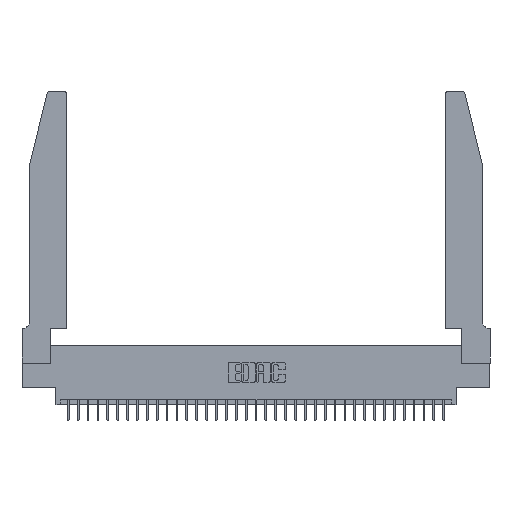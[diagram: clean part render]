
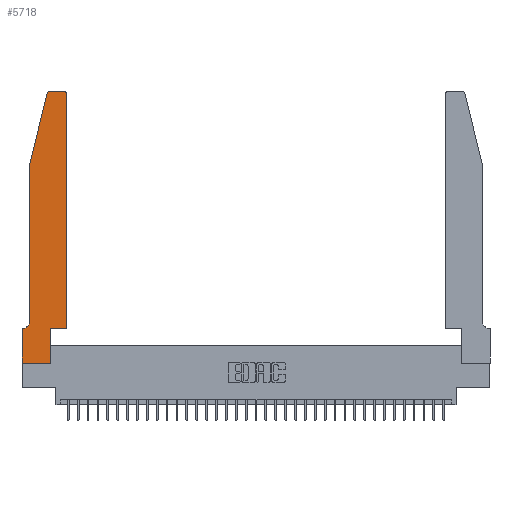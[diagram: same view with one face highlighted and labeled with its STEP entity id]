
A CAD part, top view. The second image highlights one B-rep face of the part: STEP entity #5718.
In plain terms, the highlighted planar face has unit normal (0, 0, 1).
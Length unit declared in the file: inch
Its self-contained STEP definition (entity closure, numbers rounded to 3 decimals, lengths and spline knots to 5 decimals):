
#95 = EDGE_CURVE ( 'NONE', #31149, #14235, #27200, .T. ) ;
#813 = CARTESIAN_POINT ( 'NONE',  ( 0., 0.35, 0.37 ) ) ;
#978 = CARTESIAN_POINT ( 'NONE',  ( 0.2865, 0.35, 0.37 ) ) ;
#1143 = VERTEX_POINT ( 'NONE', #2586 ) ;
#1711 = VECTOR ( 'NONE', #28622, 39.37008 ) ;
#2111 = CARTESIAN_POINT ( 'NONE',  ( 0.0755, 0.42, 0.37 ) ) ;
#2343 = CARTESIAN_POINT ( 'NONE',  ( 0., 0., 0.37 ) ) ;
#2586 = CARTESIAN_POINT ( 'NONE',  ( 0.4205, 2.75, 0.37 ) ) ;
#2658 = AXIS2_PLACEMENT_3D ( 'NONE', #31968, #15398, #34719 ) ;
#3021 = CARTESIAN_POINT ( 'NONE',  ( 0.4505, 0.35, 0.37 ) ) ;
#4048 = CARTESIAN_POINT ( 'NONE',  ( 0., 0.35, 0.37 ) ) ;
#4121 = ORIENTED_EDGE ( 'NONE', *, *, #35960, .T. ) ;
#4205 = VERTEX_POINT ( 'NONE', #33162 ) ;
#4545 = AXIS2_PLACEMENT_3D ( 'NONE', #4048, #9674, #29089 ) ;
#5190 = EDGE_CURVE ( 'NONE', #6918, #26862, #29895, .T. ) ;
#5718 = ADVANCED_FACE ( 'NONE', ( #28145 ), #23431, .T. ) ;
#5786 = VECTOR ( 'NONE', #21912, 39.37008 ) ;
#5809 = CARTESIAN_POINT ( 'NONE',  ( 0.4205, 2.72, 0.37 ) ) ;
#5863 = LINE ( 'NONE', #28262, #19833 ) ;
#6918 = VERTEX_POINT ( 'NONE', #2111 ) ;
#7825 = CIRCLE ( 'NONE', #2658, 0.03 ) ;
#8648 = DIRECTION ( 'NONE',  ( 1., 0., 0. ) ) ;
#8929 = LINE ( 'NONE', #9425, #29325 ) ;
#9186 = LINE ( 'NONE', #15319, #24863 ) ;
#9215 = CARTESIAN_POINT ( 'NONE',  ( 0., 0., 0.37 ) ) ;
#9425 = CARTESIAN_POINT ( 'NONE',  ( 0.4505, 0.35, 0.37 ) ) ;
#9674 = DIRECTION ( 'NONE',  ( 0., 0., 1. ) ) ;
#10870 = ORIENTED_EDGE ( 'NONE', *, *, #11016, .T. ) ;
#11016 = EDGE_CURVE ( 'NONE', #16986, #30710, #35275, .T. ) ;
#11626 = LINE ( 'NONE', #18405, #32845 ) ;
#12238 = DIRECTION ( 'NONE',  ( 1., 0., 0. ) ) ;
#12342 = EDGE_CURVE ( 'NONE', #30710, #21502, #28571, .T. ) ;
#12428 = VECTOR ( 'NONE', #19741, 39.37008 ) ;
#12809 = ORIENTED_EDGE ( 'NONE', *, *, #17404, .T. ) ;
#13432 = CARTESIAN_POINT ( 'NONE',  ( 0.0755, 2., 0.37 ) ) ;
#13555 = CARTESIAN_POINT ( 'NONE',  ( 0.25487, 2.72718, 0.37 ) ) ;
#13995 = ORIENTED_EDGE ( 'NONE', *, *, #18791, .T. ) ;
#14128 = ORIENTED_EDGE ( 'NONE', *, *, #95, .T. ) ;
#14235 = VERTEX_POINT ( 'NONE', #31734 ) ;
#14245 = ORIENTED_EDGE ( 'NONE', *, *, #12342, .T. ) ;
#14613 = CARTESIAN_POINT ( 'NONE',  ( 0.2865, 0., 0.37 ) ) ;
#14697 = VECTOR ( 'NONE', #28741, 39.37008 ) ;
#14736 = ORIENTED_EDGE ( 'NONE', *, *, #26750, .T. ) ;
#15319 = CARTESIAN_POINT ( 'NONE',  ( 0.0755, 0.35, 0.37 ) ) ;
#15398 = DIRECTION ( 'NONE',  ( 0., 0., 1. ) ) ;
#15996 = CARTESIAN_POINT ( 'NONE',  ( 0.0055, 0.35, 0.37 ) ) ;
#16068 = CARTESIAN_POINT ( 'NONE',  ( 0.0055, 0.42, 0.37 ) ) ;
#16353 = CARTESIAN_POINT ( 'NONE',  ( 0.2865, 0.35, 0.37 ) ) ;
#16740 = EDGE_CURVE ( 'NONE', #26862, #30041, #9186, .T. ) ;
#16756 = AXIS2_PLACEMENT_3D ( 'NONE', #5809, #25304, #8648 ) ;
#16986 = VERTEX_POINT ( 'NONE', #2343 ) ;
#17404 = EDGE_CURVE ( 'NONE', #4205, #26925, #7825, .T. ) ;
#18153 = LINE ( 'NONE', #18286, #32005 ) ;
#18220 = DIRECTION ( 'NONE',  ( -1., 0., 0. ) ) ;
#18286 = CARTESIAN_POINT ( 'NONE',  ( 0.2605, 2.75, 0.37 ) ) ;
#18405 = CARTESIAN_POINT ( 'NONE',  ( 0.0755, 2., 0.37 ) ) ;
#18791 = EDGE_CURVE ( 'NONE', #14235, #1143, #33930, .T. ) ;
#18844 = DIRECTION ( 'NONE',  ( -1., 0., 0. ) ) ;
#18991 = CARTESIAN_POINT ( 'NONE',  ( 0., 0., 0.37 ) ) ;
#19211 = CARTESIAN_POINT ( 'NONE',  ( 0.4505, 0.35, 0.37 ) ) ;
#19741 = DIRECTION ( 'NONE',  ( 0., 1., 0. ) ) ;
#19833 = VECTOR ( 'NONE', #31034, 39.37008 ) ;
#21074 = DIRECTION ( 'NONE',  ( -1., 0., 0. ) ) ;
#21502 = VERTEX_POINT ( 'NONE', #16353 ) ;
#21912 = DIRECTION ( 'NONE',  ( 1., 0., 0. ) ) ;
#23431 = PLANE ( 'NONE',  #4545 ) ;
#24863 = VECTOR ( 'NONE', #18220, 39.37008 ) ;
#25262 = ORIENTED_EDGE ( 'NONE', *, *, #5190, .T. ) ;
#25304 = DIRECTION ( 'NONE',  ( 0., 0., 1. ) ) ;
#26750 = EDGE_CURVE ( 'NONE', #1143, #4205, #18153, .T. ) ;
#26862 = VERTEX_POINT ( 'NONE', #15996 ) ;
#26925 = VERTEX_POINT ( 'NONE', #13555 ) ;
#27200 = LINE ( 'NONE', #3021, #12428 ) ;
#28145 = FACE_OUTER_BOUND ( 'NONE', #33142, .T. ) ;
#28262 = CARTESIAN_POINT ( 'NONE',  ( 0.0755, 2., 0.37 ) ) ;
#28571 = LINE ( 'NONE', #978, #14697 ) ;
#28622 = DIRECTION ( 'NONE',  ( 0., -1., 0. ) ) ;
#28741 = DIRECTION ( 'NONE',  ( 0., 1., 0. ) ) ;
#28819 = VERTEX_POINT ( 'NONE', #13432 ) ;
#28957 = ORIENTED_EDGE ( 'NONE', *, *, #34932, .T. ) ;
#29077 = AXIS2_PLACEMENT_3D ( 'NONE', #16068, #35370, #18844 ) ;
#29089 = DIRECTION ( 'NONE',  ( 1., 0., 0. ) ) ;
#29325 = VECTOR ( 'NONE', #12238, 39.37008 ) ;
#29895 = CIRCLE ( 'NONE', #29077, 0.07 ) ;
#30041 = VERTEX_POINT ( 'NONE', #813 ) ;
#30457 = LINE ( 'NONE', #9215, #1711 ) ;
#30536 = ORIENTED_EDGE ( 'NONE', *, *, #16740, .T. ) ;
#30710 = VERTEX_POINT ( 'NONE', #14613 ) ;
#31034 = DIRECTION ( 'NONE',  ( 0., -1., 0. ) ) ;
#31149 = VERTEX_POINT ( 'NONE', #19211 ) ;
#31424 = EDGE_CURVE ( 'NONE', #30041, #16986, #30457, .T. ) ;
#31707 = ORIENTED_EDGE ( 'NONE', *, *, #31424, .T. ) ;
#31734 = CARTESIAN_POINT ( 'NONE',  ( 0.4505, 2.72, 0.37 ) ) ;
#31968 = CARTESIAN_POINT ( 'NONE',  ( 0.284, 2.72, 0.37 ) ) ;
#32005 = VECTOR ( 'NONE', #21074, 39.37008 ) ;
#32845 = VECTOR ( 'NONE', #34928, 39.37008 ) ;
#33142 = EDGE_LOOP ( 'NONE', ( #14736, #12809, #28957, #33213, #25262, #30536, #31707, #10870, #14245, #4121, #14128, #13995 ) ) ;
#33162 = CARTESIAN_POINT ( 'NONE',  ( 0.284, 2.75, 0.37 ) ) ;
#33213 = ORIENTED_EDGE ( 'NONE', *, *, #35784, .T. ) ;
#33930 = CIRCLE ( 'NONE', #16756, 0.03 ) ;
#34719 = DIRECTION ( 'NONE',  ( 1., 0., 0. ) ) ;
#34928 = DIRECTION ( 'NONE',  ( -0.239, -0.971, 0. ) ) ;
#34932 = EDGE_CURVE ( 'NONE', #26925, #28819, #11626, .T. ) ;
#35275 = LINE ( 'NONE', #18991, #5786 ) ;
#35370 = DIRECTION ( 'NONE',  ( 0., 0., -1. ) ) ;
#35784 = EDGE_CURVE ( 'NONE', #28819, #6918, #5863, .T. ) ;
#35960 = EDGE_CURVE ( 'NONE', #21502, #31149, #8929, .T. ) ;
